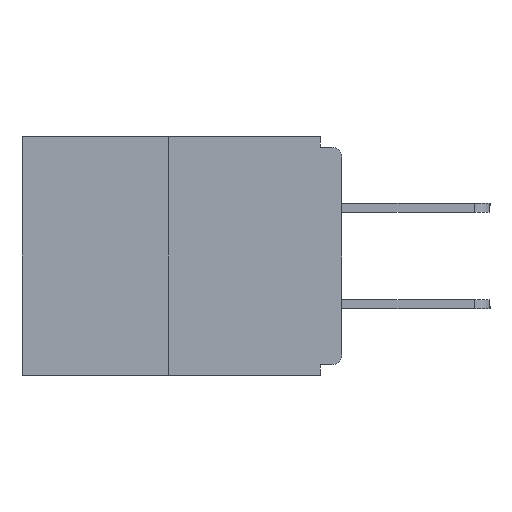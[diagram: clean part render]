
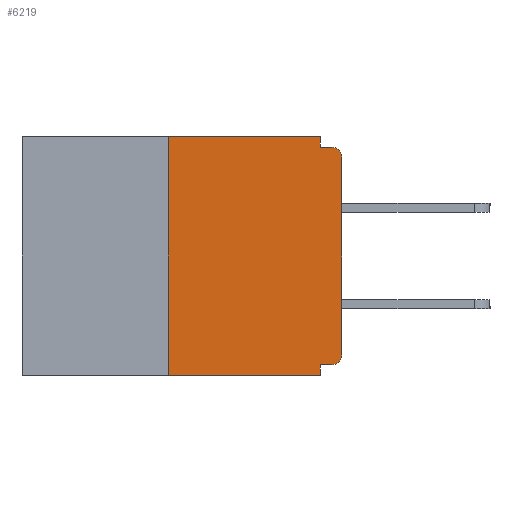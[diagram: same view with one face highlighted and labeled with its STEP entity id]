
A CAD part, left-side view. The second image highlights one B-rep face of the part: STEP entity #6219.
In plain terms, the highlighted planar face has unit normal (-1, 0, 0).
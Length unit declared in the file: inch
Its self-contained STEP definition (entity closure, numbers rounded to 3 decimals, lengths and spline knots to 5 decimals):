
#10 = ORIENTED_EDGE ( 'NONE', *, *, #2552, .F. ) ;
#367 = ORIENTED_EDGE ( 'NONE', *, *, #3374, .F. ) ;
#381 = LINE ( 'NONE', #11758, #5893 ) ;
#487 = CIRCLE ( 'NONE', #11100, 0.015 ) ;
#507 = ORIENTED_EDGE ( 'NONE', *, *, #10931, .F. ) ;
#516 = VECTOR ( 'NONE', #6874, 39.37008 ) ;
#679 = AXIS2_PLACEMENT_3D ( 'NONE', #1664, #4364, #5420 ) ;
#768 = LINE ( 'NONE', #8031, #1586 ) ;
#995 = DIRECTION ( 'NONE',  ( 0., 0., 1. ) ) ;
#1220 = CARTESIAN_POINT ( 'NONE',  ( 0., 0.46, -0.343 ) ) ;
#1296 = DIRECTION ( 'NONE',  ( 0., 0., -1. ) ) ;
#1446 = CARTESIAN_POINT ( 'NONE',  ( 0., 0.015, -0.313 ) ) ;
#1562 = ORIENTED_EDGE ( 'NONE', *, *, #3180, .T. ) ;
#1586 = VECTOR ( 'NONE', #8275, 39.37008 ) ;
#1664 = CARTESIAN_POINT ( 'NONE',  ( 0., 0.46, 0. ) ) ;
#1911 = CARTESIAN_POINT ( 'NONE',  ( 0., 0.031, -0.015 ) ) ;
#2010 = DIRECTION ( 'NONE',  ( 0., -1., 0. ) ) ;
#2425 = DIRECTION ( 'NONE',  ( -1., 0., 0. ) ) ;
#2552 = EDGE_CURVE ( 'NONE', #11319, #9021, #381, .T. ) ;
#2679 = VECTOR ( 'NONE', #10862, 39.37008 ) ;
#2680 = CARTESIAN_POINT ( 'NONE',  ( 0., 0.015, -0.015 ) ) ;
#2793 = LINE ( 'NONE', #3671, #8131 ) ;
#2813 = ORIENTED_EDGE ( 'NONE', *, *, #9893, .T. ) ;
#2881 = ORIENTED_EDGE ( 'NONE', *, *, #7888, .F. ) ;
#3043 = ORIENTED_EDGE ( 'NONE', *, *, #3676, .T. ) ;
#3180 = EDGE_CURVE ( 'NONE', #4001, #8001, #487, .T. ) ;
#3192 = CARTESIAN_POINT ( 'NONE',  ( 0., 0.031, -0.343 ) ) ;
#3374 = EDGE_CURVE ( 'NONE', #7749, #11319, #5343, .T. ) ;
#3671 = CARTESIAN_POINT ( 'NONE',  ( 0., 0.031, 0. ) ) ;
#3676 = EDGE_CURVE ( 'NONE', #6879, #4001, #768, .T. ) ;
#4001 = VERTEX_POINT ( 'NONE', #6850 ) ;
#4313 = EDGE_CURVE ( 'NONE', #9949, #8971, #6415, .T. ) ;
#4364 = DIRECTION ( 'NONE',  ( 1., 0., 0. ) ) ;
#4628 = ORIENTED_EDGE ( 'NONE', *, *, #4313, .F. ) ;
#4660 = CIRCLE ( 'NONE', #11923, 0.015 ) ;
#4766 = CARTESIAN_POINT ( 'NONE',  ( 0., 0.031, -0.328 ) ) ;
#4835 = CARTESIAN_POINT ( 'NONE',  ( 0., 0., -0.313 ) ) ;
#5236 = PLANE ( 'NONE',  #679 ) ;
#5343 = LINE ( 'NONE', #5538, #7178 ) ;
#5420 = DIRECTION ( 'NONE',  ( 0., 0., -1. ) ) ;
#5538 = CARTESIAN_POINT ( 'NONE',  ( 0., 0., -0.328 ) ) ;
#5793 = DIRECTION ( 'NONE',  ( -1., 0., 0. ) ) ;
#5837 = LINE ( 'NONE', #7626, #10876 ) ;
#5893 = VECTOR ( 'NONE', #10720, 39.37008 ) ;
#6022 = CARTESIAN_POINT ( 'NONE',  ( 0., 0.031, 0. ) ) ;
#6219 = ADVANCED_FACE ( 'NONE', ( #9186 ), #5236, .F. ) ;
#6402 = VECTOR ( 'NONE', #995, 39.37008 ) ;
#6415 = LINE ( 'NONE', #9432, #6402 ) ;
#6850 = CARTESIAN_POINT ( 'NONE',  ( 0., 0., -0.03 ) ) ;
#6874 = DIRECTION ( 'NONE',  ( 0., -1., 0. ) ) ;
#6879 = VERTEX_POINT ( 'NONE', #4835 ) ;
#7114 = CARTESIAN_POINT ( 'NONE',  ( 0., 0.46, 0. ) ) ;
#7178 = VECTOR ( 'NONE', #10073, 39.37008 ) ;
#7626 = CARTESIAN_POINT ( 'NONE',  ( 0., 0., -0.015 ) ) ;
#7676 = VERTEX_POINT ( 'NONE', #6022 ) ;
#7688 = EDGE_CURVE ( 'NONE', #9949, #9021, #10680, .T. ) ;
#7749 = VERTEX_POINT ( 'NONE', #9821 ) ;
#7888 = EDGE_CURVE ( 'NONE', #8971, #7676, #8979, .T. ) ;
#8001 = VERTEX_POINT ( 'NONE', #2680 ) ;
#8031 = CARTESIAN_POINT ( 'NONE',  ( 0., 0., 0. ) ) ;
#8094 = DIRECTION ( 'NONE',  ( 0., 0., -1. ) ) ;
#8131 = VECTOR ( 'NONE', #11038, 39.37008 ) ;
#8275 = DIRECTION ( 'NONE',  ( 0., 0., 1. ) ) ;
#8971 = VERTEX_POINT ( 'NONE', #11804 ) ;
#8979 = LINE ( 'NONE', #7114, #2679 ) ;
#9018 = EDGE_LOOP ( 'NONE', ( #2881, #4628, #10060, #10, #367, #2813, #3043, #1562, #507, #9418 ) ) ;
#9021 = VERTEX_POINT ( 'NONE', #3192 ) ;
#9186 = FACE_OUTER_BOUND ( 'NONE', #9018, .T. ) ;
#9418 = ORIENTED_EDGE ( 'NONE', *, *, #11195, .F. ) ;
#9432 = CARTESIAN_POINT ( 'NONE',  ( 0., 0.25, 0. ) ) ;
#9821 = CARTESIAN_POINT ( 'NONE',  ( 0., 0.015, -0.328 ) ) ;
#9893 = EDGE_CURVE ( 'NONE', #7749, #6879, #4660, .T. ) ;
#9949 = VERTEX_POINT ( 'NONE', #11593 ) ;
#10060 = ORIENTED_EDGE ( 'NONE', *, *, #7688, .T. ) ;
#10073 = DIRECTION ( 'NONE',  ( 0., 1., 0. ) ) ;
#10402 = CARTESIAN_POINT ( 'NONE',  ( 0., 0.015, -0.03 ) ) ;
#10459 = VERTEX_POINT ( 'NONE', #1911 ) ;
#10680 = LINE ( 'NONE', #1220, #516 ) ;
#10720 = DIRECTION ( 'NONE',  ( 0., 0., -1. ) ) ;
#10862 = DIRECTION ( 'NONE',  ( 0., -1., 0. ) ) ;
#10876 = VECTOR ( 'NONE', #2010, 39.37008 ) ;
#10931 = EDGE_CURVE ( 'NONE', #10459, #8001, #5837, .T. ) ;
#11038 = DIRECTION ( 'NONE',  ( 0., 0., -1. ) ) ;
#11100 = AXIS2_PLACEMENT_3D ( 'NONE', #10402, #5793, #1296 ) ;
#11195 = EDGE_CURVE ( 'NONE', #7676, #10459, #2793, .T. ) ;
#11319 = VERTEX_POINT ( 'NONE', #4766 ) ;
#11593 = CARTESIAN_POINT ( 'NONE',  ( 0., 0.25, -0.343 ) ) ;
#11758 = CARTESIAN_POINT ( 'NONE',  ( 0., 0.031, -0.343 ) ) ;
#11804 = CARTESIAN_POINT ( 'NONE',  ( 0., 0.25, 0. ) ) ;
#11923 = AXIS2_PLACEMENT_3D ( 'NONE', #1446, #2425, #8094 ) ;
